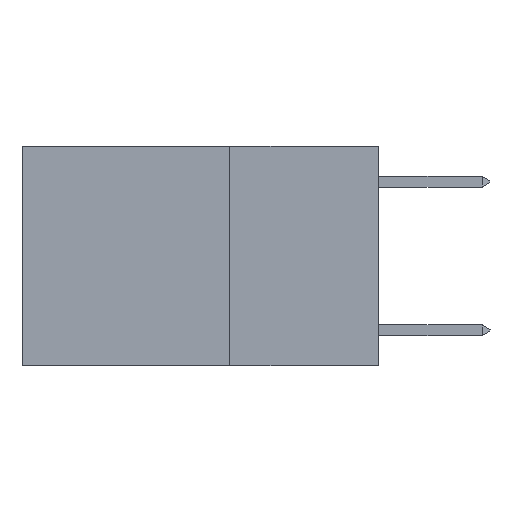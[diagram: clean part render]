
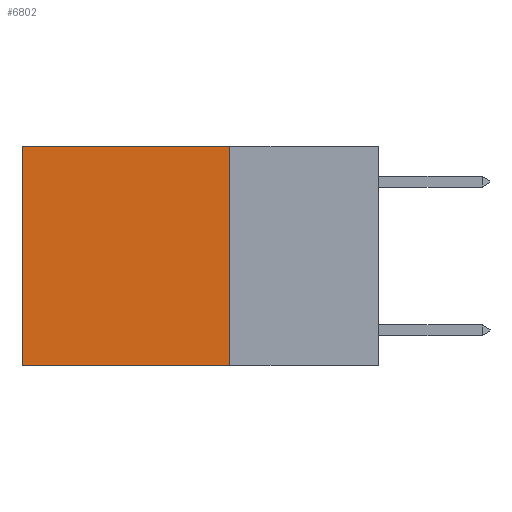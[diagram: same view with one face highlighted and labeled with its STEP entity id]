
A CAD part, left-side view. The second image highlights one B-rep face of the part: STEP entity #6802.
In plain terms, the highlighted planar face has unit normal (-1, 0, 0).
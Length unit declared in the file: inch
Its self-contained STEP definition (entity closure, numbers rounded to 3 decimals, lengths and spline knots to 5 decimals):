
#613 = PLANE ( 'NONE',  #9573 ) ;
#732 = LINE ( 'NONE', #9165, #1669 ) ;
#1669 = VECTOR ( 'NONE', #6580, 39.37008 ) ;
#1721 = FACE_OUTER_BOUND ( 'NONE', #3576, .T. ) ;
#1793 = ORIENTED_EDGE ( 'NONE', *, *, #7368, .T. ) ;
#3054 = EDGE_CURVE ( 'NONE', #4803, #10608, #732, .T. ) ;
#3483 = DIRECTION ( 'NONE',  ( 0., 0., -1. ) ) ;
#3576 = EDGE_LOOP ( 'NONE', ( #7481, #10826, #5109, #1793 ) ) ;
#4005 = CARTESIAN_POINT ( 'NONE',  ( 0.2625, 0.25, -0.37 ) ) ;
#4039 = DIRECTION ( 'NONE',  ( 0., 0., -1. ) ) ;
#4352 = DIRECTION ( 'NONE',  ( 0., 0., -1. ) ) ;
#4803 = VERTEX_POINT ( 'NONE', #4005 ) ;
#4924 = CARTESIAN_POINT ( 'NONE',  ( 0.2625, 0.25, 0. ) ) ;
#5109 = ORIENTED_EDGE ( 'NONE', *, *, #11039, .F. ) ;
#5189 = CARTESIAN_POINT ( 'NONE',  ( 0.2625, 0.25, 0. ) ) ;
#5191 = CARTESIAN_POINT ( 'NONE',  ( 0.2625, 0.6, 0. ) ) ;
#5557 = CARTESIAN_POINT ( 'NONE',  ( 0.2625, 0.6, 0. ) ) ;
#6008 = VERTEX_POINT ( 'NONE', #10144 ) ;
#6399 = VECTOR ( 'NONE', #10438, 39.37008 ) ;
#6409 = VECTOR ( 'NONE', #3483, 39.37008 ) ;
#6519 = LINE ( 'NONE', #5189, #6399 ) ;
#6580 = DIRECTION ( 'NONE',  ( 0., 1., 0. ) ) ;
#6802 = ADVANCED_FACE ( 'NONE', ( #1721 ), #613, .F. ) ;
#6860 = VECTOR ( 'NONE', #4352, 39.37008 ) ;
#7011 = EDGE_CURVE ( 'NONE', #10466, #10608, #11125, .T. ) ;
#7368 = EDGE_CURVE ( 'NONE', #6008, #10466, #6519, .T. ) ;
#7409 = DIRECTION ( 'NONE',  ( 1., 0., 0. ) ) ;
#7481 = ORIENTED_EDGE ( 'NONE', *, *, #7011, .T. ) ;
#8088 = LINE ( 'NONE', #4924, #6860 ) ;
#8366 = CARTESIAN_POINT ( 'NONE',  ( 0.2625, 0.25, 0. ) ) ;
#9165 = CARTESIAN_POINT ( 'NONE',  ( 0.2625, 0.25, -0.37 ) ) ;
#9573 = AXIS2_PLACEMENT_3D ( 'NONE', #8366, #7409, #4039 ) ;
#9782 = CARTESIAN_POINT ( 'NONE',  ( 0.2625, 0.6, -0.37 ) ) ;
#10144 = CARTESIAN_POINT ( 'NONE',  ( 0.2625, 0.25, 0. ) ) ;
#10438 = DIRECTION ( 'NONE',  ( 0., 1., 0. ) ) ;
#10466 = VERTEX_POINT ( 'NONE', #5557 ) ;
#10608 = VERTEX_POINT ( 'NONE', #9782 ) ;
#10826 = ORIENTED_EDGE ( 'NONE', *, *, #3054, .F. ) ;
#11039 = EDGE_CURVE ( 'NONE', #6008, #4803, #8088, .T. ) ;
#11125 = LINE ( 'NONE', #5191, #6409 ) ;
